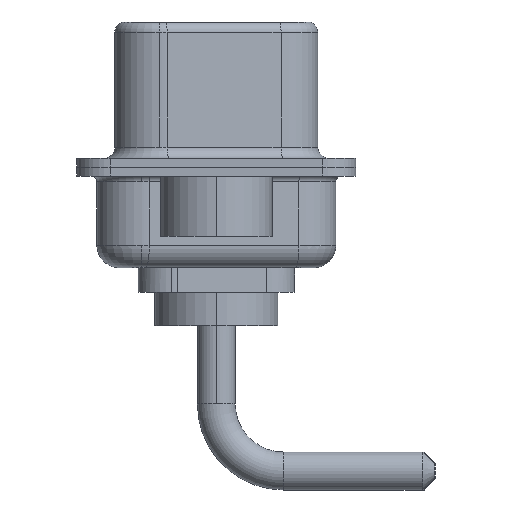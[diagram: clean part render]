
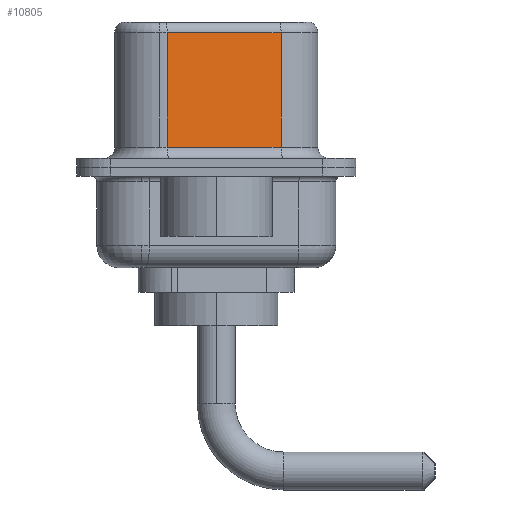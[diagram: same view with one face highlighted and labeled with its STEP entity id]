
A CAD part, left-side view. The second image highlights one B-rep face of the part: STEP entity #10805.
In plain terms, the highlighted planar face has unit normal (-0.985, -0.174, 0).
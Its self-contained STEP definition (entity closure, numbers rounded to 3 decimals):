
#313 = ORIENTED_EDGE ( 'NONE', *, *, #3940, .T. ) ;
#502 = VECTOR ( 'NONE', #4480, 1000. ) ;
#575 = LINE ( 'NONE', #9077, #11028 ) ;
#620 = LINE ( 'NONE', #1791, #8079 ) ;
#1791 = CARTESIAN_POINT ( 'NONE',  ( 4.58, -2.897, 0.9 ) ) ;
#2143 = CARTESIAN_POINT ( 'NONE',  ( 4.58, -2.897, 6.52 ) ) ;
#3041 = CARTESIAN_POINT ( 'NONE',  ( 4.58, -2.897, 6.02 ) ) ;
#3580 = DIRECTION ( 'NONE',  ( 0., 0., -1. ) ) ;
#3940 = EDGE_CURVE ( 'NONE', #9811, #11157, #575, .T. ) ;
#4157 = DIRECTION ( 'NONE',  ( 0.985, 0.174, 0. ) ) ;
#4480 = DIRECTION ( 'NONE',  ( 0., 0., -1. ) ) ;
#4577 = EDGE_CURVE ( 'NONE', #12970, #9811, #8544, .T. ) ;
#5025 = VECTOR ( 'NONE', #5292, 1000. ) ;
#5062 = DIRECTION ( 'NONE',  ( 0.174, -0.985, 0. ) ) ;
#5142 = CARTESIAN_POINT ( 'NONE',  ( 4.58, -2.897, 6.02 ) ) ;
#5292 = DIRECTION ( 'NONE',  ( -0.174, 0.985, 0. ) ) ;
#6102 = FACE_OUTER_BOUND ( 'NONE', #12522, .T. ) ;
#6332 = VERTEX_POINT ( 'NONE', #11208 ) ;
#8079 = VECTOR ( 'NONE', #5062, 1000. ) ;
#8544 = LINE ( 'NONE', #3041, #5025 ) ;
#8996 = EDGE_CURVE ( 'NONE', #11157, #6332, #620, .T. ) ;
#9077 = CARTESIAN_POINT ( 'NONE',  ( 3.68, 2.203, 6.52 ) ) ;
#9283 = AXIS2_PLACEMENT_3D ( 'NONE', #11699, #4157, #9711 ) ;
#9678 = CARTESIAN_POINT ( 'NONE',  ( 3.68, 2.203, 0.9 ) ) ;
#9711 = DIRECTION ( 'NONE',  ( -0.174, 0.985, 0. ) ) ;
#9811 = VERTEX_POINT ( 'NONE', #13755 ) ;
#10805 = ADVANCED_FACE ( 'NONE', ( #6102 ), #14192, .F. ) ;
#11028 = VECTOR ( 'NONE', #3580, 1000. ) ;
#11157 = VERTEX_POINT ( 'NONE', #9678 ) ;
#11208 = CARTESIAN_POINT ( 'NONE',  ( 4.58, -2.897, 0.9 ) ) ;
#11572 = ORIENTED_EDGE ( 'NONE', *, *, #13649, .F. ) ;
#11699 = CARTESIAN_POINT ( 'NONE',  ( 4.58, -2.897, 6.52 ) ) ;
#11722 = ORIENTED_EDGE ( 'NONE', *, *, #8996, .T. ) ;
#11964 = ORIENTED_EDGE ( 'NONE', *, *, #4577, .T. ) ;
#12522 = EDGE_LOOP ( 'NONE', ( #11572, #11964, #313, #11722 ) ) ;
#12970 = VERTEX_POINT ( 'NONE', #5142 ) ;
#13649 = EDGE_CURVE ( 'NONE', #12970, #6332, #14240, .T. ) ;
#13755 = CARTESIAN_POINT ( 'NONE',  ( 3.68, 2.203, 6.02 ) ) ;
#14192 = PLANE ( 'NONE',  #9283 ) ;
#14240 = LINE ( 'NONE', #2143, #502 ) ;
